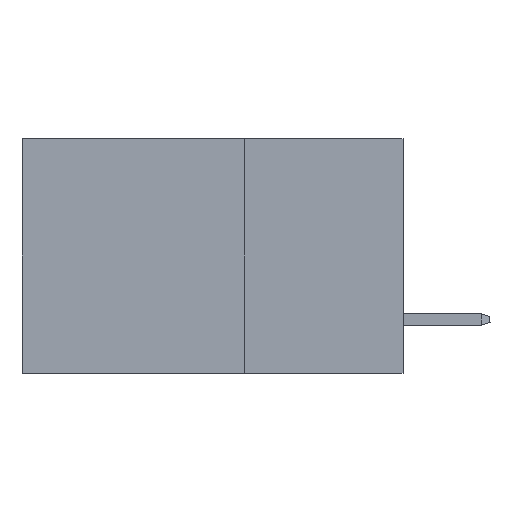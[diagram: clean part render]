
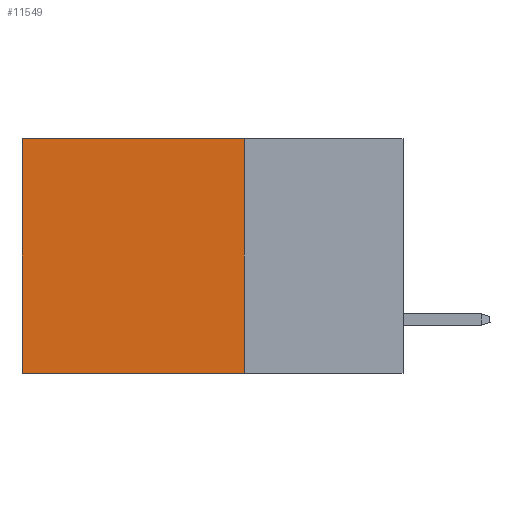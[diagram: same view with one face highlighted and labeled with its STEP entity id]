
A CAD part, left-side view. The second image highlights one B-rep face of the part: STEP entity #11549.
In plain terms, the highlighted planar face has unit normal (-1, 0, 0).
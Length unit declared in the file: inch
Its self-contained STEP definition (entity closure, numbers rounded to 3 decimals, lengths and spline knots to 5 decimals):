
#483 = LINE ( 'NONE', #23042, #10601 ) ;
#1414 = AXIS2_PLACEMENT_3D ( 'NONE', #14677, #22144, #18719 ) ;
#2876 = LINE ( 'NONE', #23898, #6146 ) ;
#3189 = ORIENTED_EDGE ( 'NONE', *, *, #16846, .T. ) ;
#5446 = PLANE ( 'NONE',  #1414 ) ;
#6146 = VECTOR ( 'NONE', #12196, 39.37008 ) ;
#6666 = VERTEX_POINT ( 'NONE', #8243 ) ;
#6935 = DIRECTION ( 'NONE',  ( 0., 1., 0. ) ) ;
#8243 = CARTESIAN_POINT ( 'NONE',  ( 0.2875, 0.6, 0. ) ) ;
#9029 = FACE_OUTER_BOUND ( 'NONE', #17782, .T. ) ;
#10601 = VECTOR ( 'NONE', #6935, 39.37008 ) ;
#11325 = EDGE_CURVE ( 'NONE', #6666, #18147, #2876, .T. ) ;
#11549 = ADVANCED_FACE ( 'NONE', ( #9029 ), #5446, .F. ) ;
#12177 = CARTESIAN_POINT ( 'NONE',  ( 0.2875, 0.25, -0.37 ) ) ;
#12196 = DIRECTION ( 'NONE',  ( 0., 0., -1. ) ) ;
#12959 = DIRECTION ( 'NONE',  ( 0., 1., 0. ) ) ;
#13693 = EDGE_CURVE ( 'NONE', #21592, #17298, #23047, .T. ) ;
#14677 = CARTESIAN_POINT ( 'NONE',  ( 0.2875, 0.25, 0. ) ) ;
#14807 = CARTESIAN_POINT ( 'NONE',  ( 0.2875, 0.25, -0.37 ) ) ;
#15229 = CARTESIAN_POINT ( 'NONE',  ( 0.2875, 0.25, 0. ) ) ;
#15744 = EDGE_CURVE ( 'NONE', #17298, #18147, #20179, .T. ) ;
#16846 = EDGE_CURVE ( 'NONE', #21592, #6666, #483, .T. ) ;
#17260 = VECTOR ( 'NONE', #22811, 39.37008 ) ;
#17298 = VERTEX_POINT ( 'NONE', #12177 ) ;
#17616 = CARTESIAN_POINT ( 'NONE',  ( 0.2875, 0.25, 0. ) ) ;
#17782 = EDGE_LOOP ( 'NONE', ( #23229, #19953, #21982, #3189 ) ) ;
#18147 = VERTEX_POINT ( 'NONE', #23167 ) ;
#18719 = DIRECTION ( 'NONE',  ( 0., 0., -1. ) ) ;
#19953 = ORIENTED_EDGE ( 'NONE', *, *, #15744, .F. ) ;
#20179 = LINE ( 'NONE', #14807, #22337 ) ;
#21592 = VERTEX_POINT ( 'NONE', #17616 ) ;
#21982 = ORIENTED_EDGE ( 'NONE', *, *, #13693, .F. ) ;
#22144 = DIRECTION ( 'NONE',  ( 1., 0., 0. ) ) ;
#22337 = VECTOR ( 'NONE', #12959, 39.37008 ) ;
#22811 = DIRECTION ( 'NONE',  ( 0., 0., -1. ) ) ;
#23042 = CARTESIAN_POINT ( 'NONE',  ( 0.2875, 0.25, 0. ) ) ;
#23047 = LINE ( 'NONE', #15229, #17260 ) ;
#23167 = CARTESIAN_POINT ( 'NONE',  ( 0.2875, 0.6, -0.37 ) ) ;
#23229 = ORIENTED_EDGE ( 'NONE', *, *, #11325, .T. ) ;
#23898 = CARTESIAN_POINT ( 'NONE',  ( 0.2875, 0.6, 0. ) ) ;
